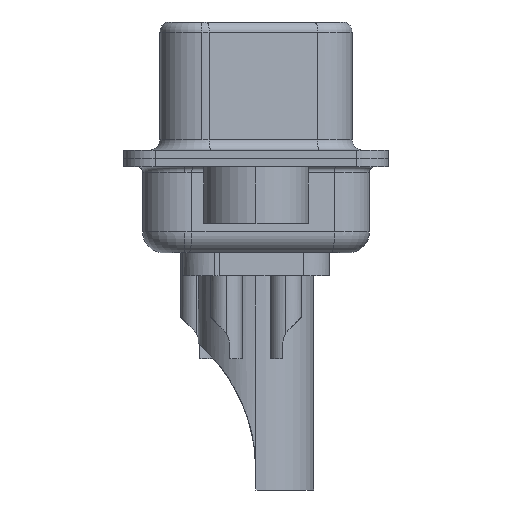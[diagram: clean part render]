
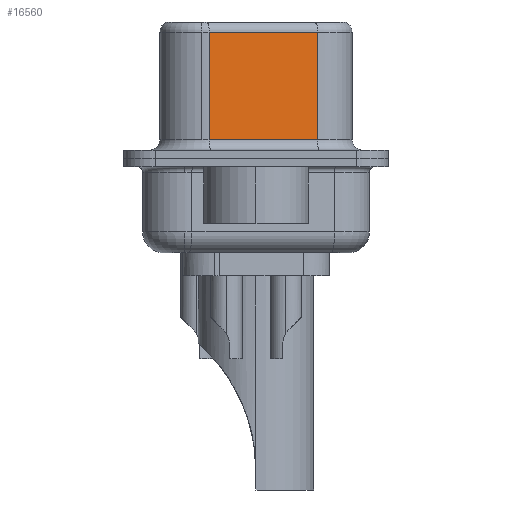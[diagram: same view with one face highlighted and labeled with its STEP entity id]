
A CAD part, left-side view. The second image highlights one B-rep face of the part: STEP entity #16560.
In plain terms, the highlighted planar face has unit normal (-0.985, -0.174, 0).
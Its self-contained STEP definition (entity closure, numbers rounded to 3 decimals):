
#428 = CARTESIAN_POINT ( 'NONE',  ( 4.585, -2.927, 6.02 ) ) ;
#1000 = ORIENTED_EDGE ( 'NONE', *, *, #17801, .T. ) ;
#1031 = DIRECTION ( 'NONE',  ( 0.174, -0.985, 0. ) ) ;
#2270 = LINE ( 'NONE', #428, #6597 ) ;
#3015 = PLANE ( 'NONE',  #20463 ) ;
#3101 = ORIENTED_EDGE ( 'NONE', *, *, #19831, .T. ) ;
#4250 = CARTESIAN_POINT ( 'NONE',  ( 4.585, -2.927, 0.9 ) ) ;
#4419 = DIRECTION ( 'NONE',  ( 0.985, 0.174, 0. ) ) ;
#4636 = ORIENTED_EDGE ( 'NONE', *, *, #16846, .T. ) ;
#4867 = VERTEX_POINT ( 'NONE', #10933 ) ;
#5653 = CARTESIAN_POINT ( 'NONE',  ( 3.675, 2.233, 6.52 ) ) ;
#6194 = EDGE_CURVE ( 'NONE', #17924, #4867, #7574, .T. ) ;
#6597 = VECTOR ( 'NONE', #13072, 1000. ) ;
#6891 = VERTEX_POINT ( 'NONE', #18145 ) ;
#7336 = EDGE_LOOP ( 'NONE', ( #8453, #4636, #1000, #3101 ) ) ;
#7574 = LINE ( 'NONE', #14359, #7839 ) ;
#7839 = VECTOR ( 'NONE', #10974, 1000. ) ;
#8453 = ORIENTED_EDGE ( 'NONE', *, *, #6194, .F. ) ;
#9024 = VERTEX_POINT ( 'NONE', #18082 ) ;
#10933 = CARTESIAN_POINT ( 'NONE',  ( 4.585, -2.927, 0.9 ) ) ;
#10974 = DIRECTION ( 'NONE',  ( 0., 0., -1. ) ) ;
#11089 = DIRECTION ( 'NONE',  ( -0.174, 0.985, 0. ) ) ;
#11192 = CARTESIAN_POINT ( 'NONE',  ( 4.585, -2.927, 6.02 ) ) ;
#13072 = DIRECTION ( 'NONE',  ( -0.174, 0.985, 0. ) ) ;
#13590 = DIRECTION ( 'NONE',  ( 0., 0., -1. ) ) ;
#14260 = CARTESIAN_POINT ( 'NONE',  ( 4.585, -2.927, 6.52 ) ) ;
#14359 = CARTESIAN_POINT ( 'NONE',  ( 4.585, -2.927, 6.52 ) ) ;
#15820 = VECTOR ( 'NONE', #1031, 1000. ) ;
#16560 = ADVANCED_FACE ( 'NONE', ( #20415 ), #3015, .F. ) ;
#16846 = EDGE_CURVE ( 'NONE', #17924, #6891, #2270, .T. ) ;
#17801 = EDGE_CURVE ( 'NONE', #6891, #9024, #19401, .T. ) ;
#17924 = VERTEX_POINT ( 'NONE', #11192 ) ;
#18082 = CARTESIAN_POINT ( 'NONE',  ( 3.675, 2.233, 0.9 ) ) ;
#18145 = CARTESIAN_POINT ( 'NONE',  ( 3.675, 2.233, 6.02 ) ) ;
#18870 = VECTOR ( 'NONE', #13590, 1000. ) ;
#19401 = LINE ( 'NONE', #5653, #18870 ) ;
#19831 = EDGE_CURVE ( 'NONE', #9024, #4867, #20093, .T. ) ;
#20093 = LINE ( 'NONE', #4250, #15820 ) ;
#20415 = FACE_OUTER_BOUND ( 'NONE', #7336, .T. ) ;
#20463 = AXIS2_PLACEMENT_3D ( 'NONE', #14260, #4419, #11089 ) ;
